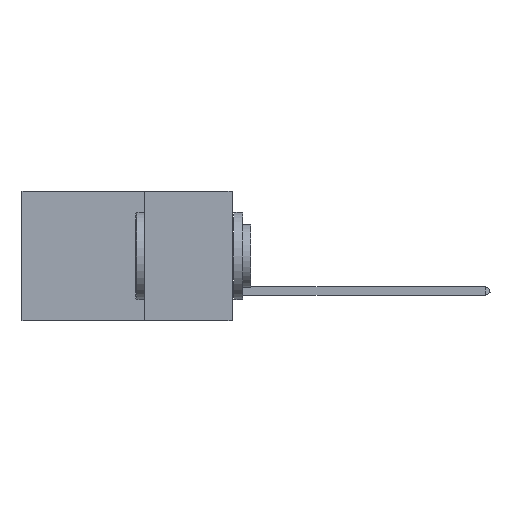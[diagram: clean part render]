
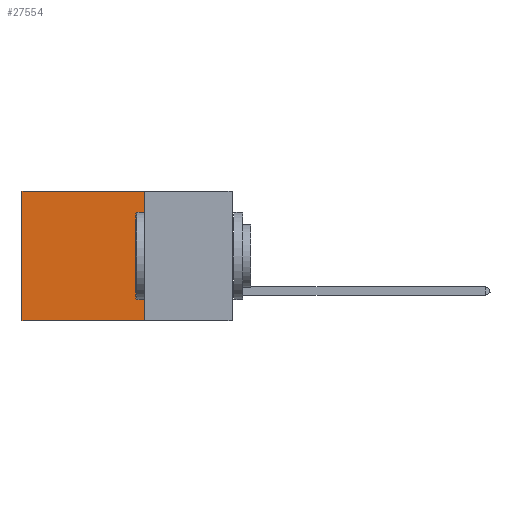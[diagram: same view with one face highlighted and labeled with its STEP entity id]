
A CAD part, left-side view. The second image highlights one B-rep face of the part: STEP entity #27554.
In plain terms, the highlighted planar face has unit normal (-1, 0, 0).
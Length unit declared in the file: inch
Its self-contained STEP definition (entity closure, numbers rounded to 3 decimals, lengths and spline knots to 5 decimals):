
#343 = CARTESIAN_POINT ( 'NONE',  ( 0.2875, 0.25, -0.37 ) ) ;
#795 = DIRECTION ( 'NONE',  ( 0., 1., 0. ) ) ;
#1099 = CARTESIAN_POINT ( 'NONE',  ( 0.2875, 0.25, 0. ) ) ;
#3470 = VECTOR ( 'NONE', #13807, 39.37008 ) ;
#3561 = CARTESIAN_POINT ( 'NONE',  ( 0.2875, 0.25, -0.37 ) ) ;
#4150 = VERTEX_POINT ( 'NONE', #343 ) ;
#5680 = DIRECTION ( 'NONE',  ( 0., 0., -1. ) ) ;
#6981 = LINE ( 'NONE', #15620, #8135 ) ;
#7825 = EDGE_LOOP ( 'NONE', ( #21549, #18144, #20847, #15895 ) ) ;
#8135 = VECTOR ( 'NONE', #5680, 39.37008 ) ;
#9422 = VERTEX_POINT ( 'NONE', #25740 ) ;
#9594 = VERTEX_POINT ( 'NONE', #19927 ) ;
#11351 = LINE ( 'NONE', #3561, #3470 ) ;
#11494 = PLANE ( 'NONE',  #23809 ) ;
#12253 = VECTOR ( 'NONE', #795, 39.37008 ) ;
#13807 = DIRECTION ( 'NONE',  ( 0., 1., 0. ) ) ;
#14716 = CARTESIAN_POINT ( 'NONE',  ( 0.2875, 0.6, 0. ) ) ;
#15620 = CARTESIAN_POINT ( 'NONE',  ( 0.2875, 0.25, 0. ) ) ;
#15895 = ORIENTED_EDGE ( 'NONE', *, *, #27968, .T. ) ;
#17003 = EDGE_CURVE ( 'NONE', #4150, #20068, #11351, .T. ) ;
#18144 = ORIENTED_EDGE ( 'NONE', *, *, #17003, .F. ) ;
#19377 = VECTOR ( 'NONE', #29191, 39.37008 ) ;
#19927 = CARTESIAN_POINT ( 'NONE',  ( 0.2875, 0.25, 0. ) ) ;
#20068 = VERTEX_POINT ( 'NONE', #29655 ) ;
#20847 = ORIENTED_EDGE ( 'NONE', *, *, #25124, .F. ) ;
#21549 = ORIENTED_EDGE ( 'NONE', *, *, #27810, .T. ) ;
#23521 = LINE ( 'NONE', #14716, #19377 ) ;
#23809 = AXIS2_PLACEMENT_3D ( 'NONE', #30660, #25671, #30259 ) ;
#25124 = EDGE_CURVE ( 'NONE', #9594, #4150, #6981, .T. ) ;
#25671 = DIRECTION ( 'NONE',  ( 1., 0., 0. ) ) ;
#25740 = CARTESIAN_POINT ( 'NONE',  ( 0.2875, 0.6, 0. ) ) ;
#27554 = ADVANCED_FACE ( 'NONE', ( #29719 ), #11494, .F. ) ;
#27810 = EDGE_CURVE ( 'NONE', #9422, #20068, #23521, .T. ) ;
#27968 = EDGE_CURVE ( 'NONE', #9594, #9422, #30605, .T. ) ;
#29191 = DIRECTION ( 'NONE',  ( 0., 0., -1. ) ) ;
#29655 = CARTESIAN_POINT ( 'NONE',  ( 0.2875, 0.6, -0.37 ) ) ;
#29719 = FACE_OUTER_BOUND ( 'NONE', #7825, .T. ) ;
#30259 = DIRECTION ( 'NONE',  ( 0., 0., -1. ) ) ;
#30605 = LINE ( 'NONE', #1099, #12253 ) ;
#30660 = CARTESIAN_POINT ( 'NONE',  ( 0.2875, 0.25, 0. ) ) ;
